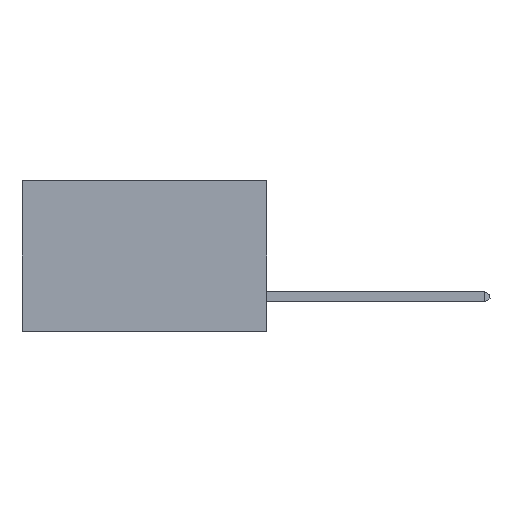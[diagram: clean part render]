
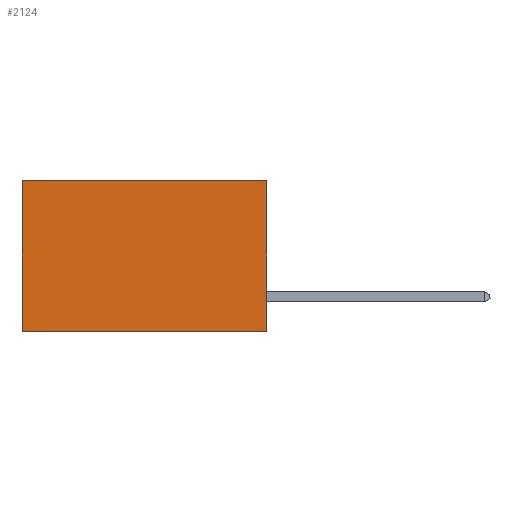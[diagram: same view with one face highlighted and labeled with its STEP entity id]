
A CAD part, left-side view. The second image highlights one B-rep face of the part: STEP entity #2124.
In plain terms, the highlighted planar face has unit normal (-1, 0, 0).
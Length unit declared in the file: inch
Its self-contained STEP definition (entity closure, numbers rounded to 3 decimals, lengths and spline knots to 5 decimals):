
#160 = ORIENTED_EDGE ( 'NONE', *, *, #2414, .T. ) ;
#167 = DIRECTION ( 'NONE',  ( 1., 0., 0. ) ) ;
#233 = DIRECTION ( 'NONE',  ( 0., 1., 0. ) ) ;
#356 = CARTESIAN_POINT ( 'NONE',  ( 0.2875, 0., 0. ) ) ;
#531 = AXIS2_PLACEMENT_3D ( 'NONE', #356, #167, #5391 ) ;
#700 = LINE ( 'NONE', #9597, #6671 ) ;
#759 = CARTESIAN_POINT ( 'NONE',  ( 0.2875, 0., -0.37 ) ) ;
#766 = ORIENTED_EDGE ( 'NONE', *, *, #4333, .F. ) ;
#1203 = ORIENTED_EDGE ( 'NONE', *, *, #5935, .T. ) ;
#1539 = VERTEX_POINT ( 'NONE', #2548 ) ;
#1704 = EDGE_CURVE ( 'NONE', #5817, #3437, #700, .T. ) ;
#2124 = ADVANCED_FACE ( 'NONE', ( #9430 ), #4415, .F. ) ;
#2414 = EDGE_CURVE ( 'NONE', #6717, #1539, #9133, .T. ) ;
#2548 = CARTESIAN_POINT ( 'NONE',  ( 0.2875, 0.6, -0.37 ) ) ;
#2910 = EDGE_LOOP ( 'NONE', ( #160, #766, #6184, #1203 ) ) ;
#3253 = VECTOR ( 'NONE', #5889, 39.37008 ) ;
#3437 = VERTEX_POINT ( 'NONE', #759 ) ;
#3732 = DIRECTION ( 'NONE',  ( 0., 0., -1. ) ) ;
#4333 = EDGE_CURVE ( 'NONE', #3437, #1539, #8809, .T. ) ;
#4415 = PLANE ( 'NONE',  #531 ) ;
#4483 = LINE ( 'NONE', #9463, #9650 ) ;
#4534 = CARTESIAN_POINT ( 'NONE',  ( 0.2875, 0., -0.37 ) ) ;
#5135 = CARTESIAN_POINT ( 'NONE',  ( 0.2875, 0.6, 0. ) ) ;
#5391 = DIRECTION ( 'NONE',  ( 0., 0., -1. ) ) ;
#5428 = CARTESIAN_POINT ( 'NONE',  ( 0.2875, 0.6, 0. ) ) ;
#5495 = DIRECTION ( 'NONE',  ( 0., 1., 0. ) ) ;
#5817 = VERTEX_POINT ( 'NONE', #9149 ) ;
#5889 = DIRECTION ( 'NONE',  ( 0., 0., -1. ) ) ;
#5935 = EDGE_CURVE ( 'NONE', #5817, #6717, #4483, .T. ) ;
#6184 = ORIENTED_EDGE ( 'NONE', *, *, #1704, .F. ) ;
#6671 = VECTOR ( 'NONE', #3732, 39.37008 ) ;
#6717 = VERTEX_POINT ( 'NONE', #5135 ) ;
#8616 = VECTOR ( 'NONE', #5495, 39.37008 ) ;
#8809 = LINE ( 'NONE', #4534, #8616 ) ;
#9133 = LINE ( 'NONE', #5428, #3253 ) ;
#9149 = CARTESIAN_POINT ( 'NONE',  ( 0.2875, 0., 0. ) ) ;
#9430 = FACE_OUTER_BOUND ( 'NONE', #2910, .T. ) ;
#9463 = CARTESIAN_POINT ( 'NONE',  ( 0.2875, 0., 0. ) ) ;
#9597 = CARTESIAN_POINT ( 'NONE',  ( 0.2875, 0., 0. ) ) ;
#9650 = VECTOR ( 'NONE', #233, 39.37008 ) ;
